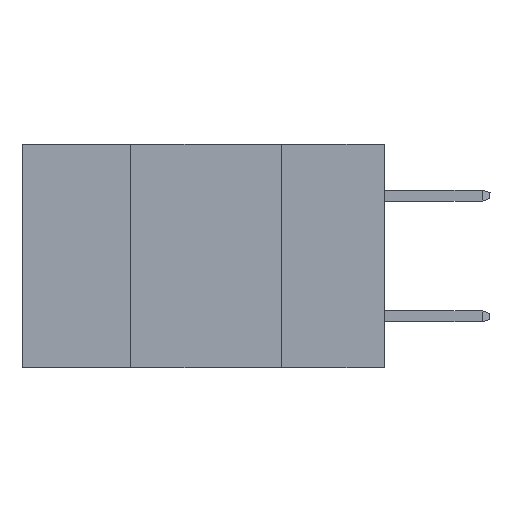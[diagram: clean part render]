
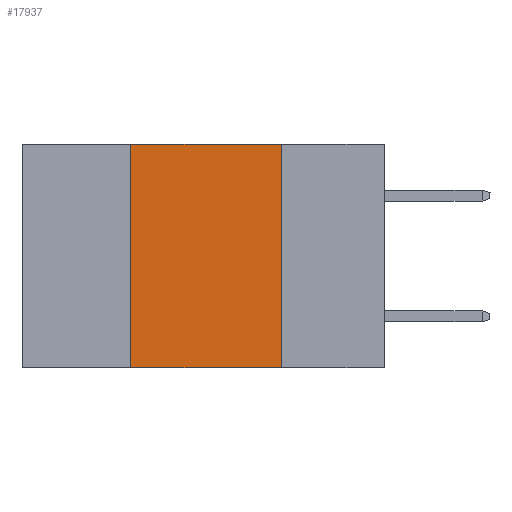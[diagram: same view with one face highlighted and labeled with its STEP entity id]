
A CAD part, left-side view. The second image highlights one B-rep face of the part: STEP entity #17937.
In plain terms, the highlighted planar face has unit normal (-1, 0, 0).
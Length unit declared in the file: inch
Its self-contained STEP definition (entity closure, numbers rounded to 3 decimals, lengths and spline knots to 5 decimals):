
#93 = VERTEX_POINT ( 'NONE', #12258 ) ;
#293 = CARTESIAN_POINT ( 'NONE',  ( 0., 0.6, -0.37 ) ) ;
#666 = EDGE_CURVE ( 'NONE', #6624, #11529, #12216, .T. ) ;
#700 = DIRECTION ( 'NONE',  ( 0., 0., -1. ) ) ;
#914 = LINE ( 'NONE', #25003, #22419 ) ;
#2562 = DIRECTION ( 'NONE',  ( 1., 0., 0. ) ) ;
#3123 = ORIENTED_EDGE ( 'NONE', *, *, #17177, .F. ) ;
#4268 = DIRECTION ( 'NONE',  ( 0., -1., 0. ) ) ;
#6624 = VERTEX_POINT ( 'NONE', #18498 ) ;
#6911 = CARTESIAN_POINT ( 'NONE',  ( 0., 0.42, 0. ) ) ;
#7626 = ORIENTED_EDGE ( 'NONE', *, *, #666, .F. ) ;
#8473 = CARTESIAN_POINT ( 'NONE',  ( 0., 0.6, 0. ) ) ;
#8847 = EDGE_CURVE ( 'NONE', #18704, #93, #914, .T. ) ;
#10185 = VECTOR ( 'NONE', #4268, 39.37008 ) ;
#11320 = FACE_OUTER_BOUND ( 'NONE', #24557, .T. ) ;
#11529 = VERTEX_POINT ( 'NONE', #23880 ) ;
#12216 = LINE ( 'NONE', #6911, #21912 ) ;
#12258 = CARTESIAN_POINT ( 'NONE',  ( 0., 0.17, -0.37 ) ) ;
#12618 = ORIENTED_EDGE ( 'NONE', *, *, #22427, .T. ) ;
#14116 = CARTESIAN_POINT ( 'NONE',  ( 0., 0.6, 0. ) ) ;
#14187 = ORIENTED_EDGE ( 'NONE', *, *, #8847, .F. ) ;
#14522 = AXIS2_PLACEMENT_3D ( 'NONE', #14116, #2562, #700 ) ;
#15337 = DIRECTION ( 'NONE',  ( 0., 0., -1. ) ) ;
#15438 = LINE ( 'NONE', #293, #20885 ) ;
#15972 = PLANE ( 'NONE',  #14522 ) ;
#16703 = CARTESIAN_POINT ( 'NONE',  ( 0., 0.17, 0. ) ) ;
#16767 = DIRECTION ( 'NONE',  ( 0., 0., 1. ) ) ;
#17177 = EDGE_CURVE ( 'NONE', #11529, #18704, #23196, .T. ) ;
#17937 = ADVANCED_FACE ( 'NONE', ( #11320 ), #15972, .F. ) ;
#18498 = CARTESIAN_POINT ( 'NONE',  ( 0., 0.42, -0.37 ) ) ;
#18704 = VERTEX_POINT ( 'NONE', #16703 ) ;
#19301 = DIRECTION ( 'NONE',  ( 0., -1., 0. ) ) ;
#20885 = VECTOR ( 'NONE', #19301, 39.37008 ) ;
#21912 = VECTOR ( 'NONE', #16767, 39.37008 ) ;
#22419 = VECTOR ( 'NONE', #15337, 39.37008 ) ;
#22427 = EDGE_CURVE ( 'NONE', #6624, #93, #15438, .T. ) ;
#23196 = LINE ( 'NONE', #8473, #10185 ) ;
#23880 = CARTESIAN_POINT ( 'NONE',  ( 0., 0.42, 0. ) ) ;
#24557 = EDGE_LOOP ( 'NONE', ( #14187, #3123, #7626, #12618 ) ) ;
#25003 = CARTESIAN_POINT ( 'NONE',  ( 0., 0.17, 0. ) ) ;
